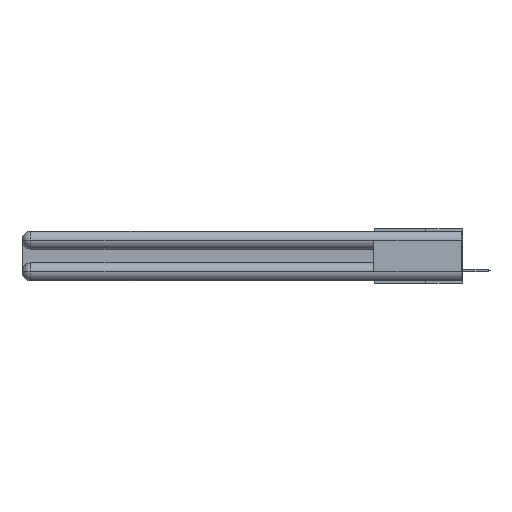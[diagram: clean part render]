
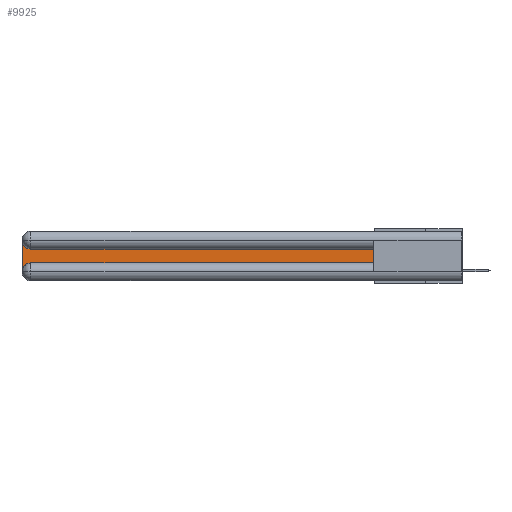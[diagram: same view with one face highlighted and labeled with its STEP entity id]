
A CAD part, left-side view. The second image highlights one B-rep face of the part: STEP entity #9925.
In plain terms, the highlighted planar face has unit normal (-1, 0, 0).
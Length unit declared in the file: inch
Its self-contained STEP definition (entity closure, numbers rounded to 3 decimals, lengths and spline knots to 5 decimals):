
#3 = CARTESIAN_POINT ( 'NONE',  ( 0.075, 0.6, -0.2175 ) ) ;
#54 = AXIS2_PLACEMENT_3D ( 'NONE', #11819, #22792, #11908 ) ;
#409 = VERTEX_POINT ( 'NONE', #23677 ) ;
#1465 = VERTEX_POINT ( 'NONE', #23820 ) ;
#1865 = DIRECTION ( 'NONE',  ( 1., 0., 0. ) ) ;
#2348 = DIRECTION ( 'NONE',  ( 0., 0., -1. ) ) ;
#2607 = CARTESIAN_POINT ( 'NONE',  ( 0.075, 0.6, -0.1225 ) ) ;
#2619 = CARTESIAN_POINT ( 'NONE',  ( 0.075, 3., -0.2175 ) ) ;
#2765 = VERTEX_POINT ( 'NONE', #22423 ) ;
#3938 = LINE ( 'NONE', #3, #14669 ) ;
#4420 = DIRECTION ( 'NONE',  ( 0., 0., -1. ) ) ;
#4511 = LINE ( 'NONE', #2619, #20907 ) ;
#4670 = EDGE_LOOP ( 'NONE', ( #22950, #12416, #15662, #22571, #6470, #21460 ) ) ;
#4826 = FACE_OUTER_BOUND ( 'NONE', #4670, .T. ) ;
#6470 = ORIENTED_EDGE ( 'NONE', *, *, #12392, .T. ) ;
#7705 = CARTESIAN_POINT ( 'NONE',  ( 0.075, 3., -0.0625 ) ) ;
#8161 = AXIS2_PLACEMENT_3D ( 'NONE', #11615, #9745, #13647 ) ;
#8578 = VERTEX_POINT ( 'NONE', #11798 ) ;
#8885 = DIRECTION ( 'NONE',  ( 0., -1., 0. ) ) ;
#9348 = CIRCLE ( 'NONE', #8161, 0.06 ) ;
#9745 = DIRECTION ( 'NONE',  ( 1., 0., 0. ) ) ;
#9760 = EDGE_CURVE ( 'NONE', #24603, #2765, #4511, .T. ) ;
#9925 = ADVANCED_FACE ( 'NONE', ( #4826 ), #11995, .F. ) ;
#10812 = DIRECTION ( 'NONE',  ( 0., 1., 0. ) ) ;
#11368 = VECTOR ( 'NONE', #8885, 39.37008 ) ;
#11615 = CARTESIAN_POINT ( 'NONE',  ( 0.075, 2.94, -0.0625 ) ) ;
#11798 = CARTESIAN_POINT ( 'NONE',  ( 0.075, 0.6, -0.2175 ) ) ;
#11819 = CARTESIAN_POINT ( 'NONE',  ( 0.075, 3., -0.1225 ) ) ;
#11908 = DIRECTION ( 'NONE',  ( 0., 0., -1. ) ) ;
#11995 = PLANE ( 'NONE',  #54 ) ;
#12392 = EDGE_CURVE ( 'NONE', #13520, #8578, #24397, .T. ) ;
#12416 = ORIENTED_EDGE ( 'NONE', *, *, #19778, .T. ) ;
#13520 = VERTEX_POINT ( 'NONE', #21201 ) ;
#13647 = DIRECTION ( 'NONE',  ( 0., 0., -1. ) ) ;
#14669 = VECTOR ( 'NONE', #19420, 39.37008 ) ;
#14935 = AXIS2_PLACEMENT_3D ( 'NONE', #23272, #1865, #4420 ) ;
#15662 = ORIENTED_EDGE ( 'NONE', *, *, #9760, .T. ) ;
#19420 = DIRECTION ( 'NONE',  ( 0., 0., 1. ) ) ;
#19778 = EDGE_CURVE ( 'NONE', #409, #24603, #9348, .T. ) ;
#19949 = VECTOR ( 'NONE', #10812, 39.37008 ) ;
#20347 = EDGE_CURVE ( 'NONE', #2765, #13520, #25743, .T. ) ;
#20614 = LINE ( 'NONE', #2607, #19949 ) ;
#20907 = VECTOR ( 'NONE', #2348, 39.37008 ) ;
#21201 = CARTESIAN_POINT ( 'NONE',  ( 0.075, 2.94, -0.2175 ) ) ;
#21329 = EDGE_CURVE ( 'NONE', #1465, #409, #20614, .T. ) ;
#21460 = ORIENTED_EDGE ( 'NONE', *, *, #24987, .T. ) ;
#21702 = CARTESIAN_POINT ( 'NONE',  ( 0.075, 0.6, -0.2175 ) ) ;
#22423 = CARTESIAN_POINT ( 'NONE',  ( 0.075, 3., -0.2775 ) ) ;
#22571 = ORIENTED_EDGE ( 'NONE', *, *, #20347, .T. ) ;
#22792 = DIRECTION ( 'NONE',  ( 1., 0., 0. ) ) ;
#22950 = ORIENTED_EDGE ( 'NONE', *, *, #21329, .T. ) ;
#23272 = CARTESIAN_POINT ( 'NONE',  ( 0.075, 2.94, -0.2775 ) ) ;
#23677 = CARTESIAN_POINT ( 'NONE',  ( 0.075, 2.94, -0.1225 ) ) ;
#23820 = CARTESIAN_POINT ( 'NONE',  ( 0.075, 0.6, -0.1225 ) ) ;
#24397 = LINE ( 'NONE', #21702, #11368 ) ;
#24603 = VERTEX_POINT ( 'NONE', #7705 ) ;
#24987 = EDGE_CURVE ( 'NONE', #8578, #1465, #3938, .T. ) ;
#25743 = CIRCLE ( 'NONE', #14935, 0.06 ) ;
